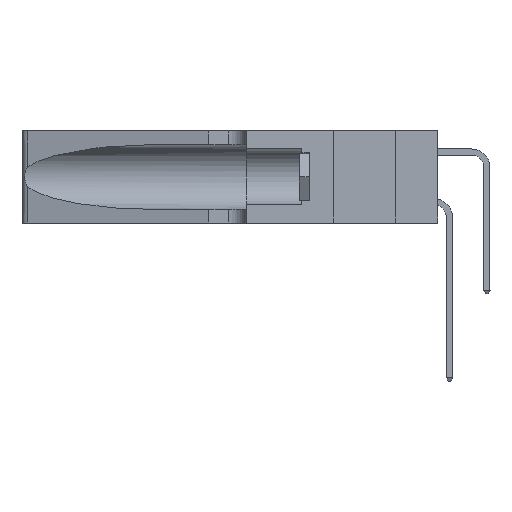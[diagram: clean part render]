
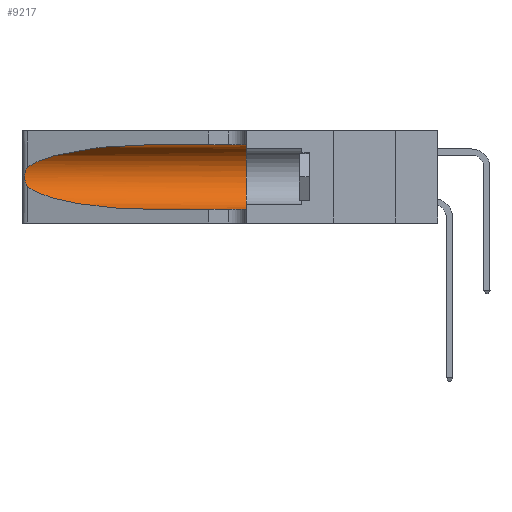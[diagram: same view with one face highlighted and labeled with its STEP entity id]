
A CAD part, left-side view. The second image highlights one B-rep face of the part: STEP entity #9217.
In plain terms, the highlighted cylindrical face has radius 3.308 mm (diameter 6.617 mm), a partial arc.
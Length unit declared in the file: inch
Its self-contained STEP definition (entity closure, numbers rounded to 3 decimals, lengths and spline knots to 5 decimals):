
#25 = VERTEX_POINT ( 'NONE', #38068 ) ;
#346 = CARTESIAN_POINT ( 'NONE',  ( 0.25487, 1.22718, 0.14631 ) ) ;
#667 = ORIENTED_EDGE ( 'NONE', *, *, #3955, .F. ) ;
#1703 = FACE_OUTER_BOUND ( 'NONE', #33231, .T. ) ;
#2833 = CARTESIAN_POINT ( 'NONE',  ( 0.25555, 1.22993, 0.14849 ) ) ;
#2927 = CARTESIAN_POINT ( 'NONE',  ( 0.2373, 1.15595, 0.08982 ) ) ;
#3357 = VERTEX_POINT ( 'NONE', #346 ) ;
#3804 = CARTESIAN_POINT ( 'NONE',  ( 0.1305, 0.72297, 0.05475 ) ) ;
#3955 = EDGE_CURVE ( 'NONE', #25, #28407, #20215, .T. ) ;
#4011 = ORIENTED_EDGE ( 'NONE', *, *, #23458, .T. ) ;
#5024 = CARTESIAN_POINT ( 'NONE',  ( 0.1305, 0.35, 0.05475 ) ) ;
#5117 = B_SPLINE_CURVE_WITH_KNOTS ( 'NONE', 3,
 ( #5623, #23829, #26789, #8834, #29805, #11863, #32823, #14911, #35775, #17950, #38713, #20964, #2833, #23957 ),
 .UNSPECIFIED., .F., .F.,
 ( 4, 2, 2, 2, 2, 2, 4 ),
 ( 0., 0.00027, 0.00053, 0.00107, 0.0016, 0.00187, 0.00214 ),
 .UNSPECIFIED. ) ;
#5476 = DIRECTION ( 'NONE',  ( 0., 0., -1. ) ) ;
#5623 = CARTESIAN_POINT ( 'NONE',  ( 0.25487, 1.22718, 0.22369 ) ) ;
#6643 = LINE ( 'NONE', #36633, #38463 ) ;
#6791 = EDGE_CURVE ( 'NONE', #25249, #28407, #6643, .T. ) ;
#7832 = CARTESIAN_POINT ( 'NONE',  ( 0.1305, 0.72297, 0.31525 ) ) ;
#8834 = CARTESIAN_POINT ( 'NONE',  ( 0.25787, 1.23484, 0.2124 ) ) ;
#9059 = CARTESIAN_POINT ( 'NONE',  ( 0.25487, 1.22718, 0.14631 ) ) ;
#9217 = ADVANCED_FACE ( 'NONE', ( #1703 ), #16909, .F. ) ;
#10066 = DIRECTION ( 'NONE',  ( 0., 1., 0. ) ) ;
#10710 = ORIENTED_EDGE ( 'NONE', *, *, #35669, .F. ) ;
#10867 = CARTESIAN_POINT ( 'NONE',  ( 0.2373, 1.15595, 0.28018 ) ) ;
#11863 = CARTESIAN_POINT ( 'NONE',  ( 0.26018, 1.23835, 0.19895 ) ) ;
#12324 = VECTOR ( 'NONE', #37208, 39.37008 ) ;
#12525 = CARTESIAN_POINT ( 'NONE',  ( 0.25487, 1.22718, 0.22369 ) ) ;
#13357 = CARTESIAN_POINT ( 'NONE',  ( 0.1305, 1.61858, 0.31525 ) ) ;
#14242 = LINE ( 'NONE', #13357, #12324 ) ;
#14911 = CARTESIAN_POINT ( 'NONE',  ( 0.26075, 1.23896, 0.178 ) ) ;
#14937 = EDGE_CURVE ( 'NONE', #23029, #3357, #5117, .T. ) ;
#16321 =( BOUNDED_CURVE ( )  B_SPLINE_CURVE ( 3, ( #7832, #28805, #10867, #31842 ),
 .UNSPECIFIED., .F., .F. ) 
 B_SPLINE_CURVE_WITH_KNOTS ( ( 4, 4 ),
 ( 1.5708, 2.84003 ),
 .UNSPECIFIED. ) 
 CURVE ( )  GEOMETRIC_REPRESENTATION_ITEM ( )  RATIONAL_B_SPLINE_CURVE ( ( 1., 0.87, 0.87, 1. ) ) 
 REPRESENTATION_ITEM ( '' )  );
#16909 = CYLINDRICAL_SURFACE ( 'NONE', #33762, 0.13025 ) ;
#17805 = CARTESIAN_POINT ( 'NONE',  ( 0.18966, 0.96281, 0.05475 ) ) ;
#17950 = CARTESIAN_POINT ( 'NONE',  ( 0.25856, 1.23593, 0.16098 ) ) ;
#18834 = DIRECTION ( 'NONE',  ( 0., -1., 0. ) ) ;
#20215 = CIRCLE ( 'NONE', #34363, 0.13025 ) ;
#20574 = DIRECTION ( 'NONE',  ( 0., -1., 0. ) ) ;
#20964 = CARTESIAN_POINT ( 'NONE',  ( 0.25639, 1.23186, 0.15144 ) ) ;
#21180 = CARTESIAN_POINT ( 'NONE',  ( 0.1305, 0.72297, 0.05475 ) ) ;
#21561 = CARTESIAN_POINT ( 'NONE',  ( 0.1305, 0.72297, 0.31525 ) ) ;
#21809 = VERTEX_POINT ( 'NONE', #21561 ) ;
#21999 = ORIENTED_EDGE ( 'NONE', *, *, #31473, .T. ) ;
#23029 = VERTEX_POINT ( 'NONE', #12525 ) ;
#23458 = EDGE_CURVE ( 'NONE', #21809, #23029, #16321, .T. ) ;
#23829 = CARTESIAN_POINT ( 'NONE',  ( 0.25555, 1.22994, 0.2215 ) ) ;
#23957 = CARTESIAN_POINT ( 'NONE',  ( 0.25487, 1.22718, 0.14631 ) ) ;
#25249 = VERTEX_POINT ( 'NONE', #3804 ) ;
#26789 = CARTESIAN_POINT ( 'NONE',  ( 0.25639, 1.23184, 0.21858 ) ) ;
#28000 = CARTESIAN_POINT ( 'NONE',  ( 0.1305, 0.35, 0.185 ) ) ;
#28027 = ORIENTED_EDGE ( 'NONE', *, *, #14937, .T. ) ;
#28407 = VERTEX_POINT ( 'NONE', #5024 ) ;
#28805 = CARTESIAN_POINT ( 'NONE',  ( 0.18966, 0.96281, 0.31525 ) ) ;
#29541 = CARTESIAN_POINT ( 'NONE',  ( 0.1305, 1.61858, 0.185 ) ) ;
#29805 = CARTESIAN_POINT ( 'NONE',  ( 0.25854, 1.2359, 0.20912 ) ) ;
#29916 = ORIENTED_EDGE ( 'NONE', *, *, #6791, .T. ) ;
#31053 = DIRECTION ( 'NONE',  ( 0., 0., 1. ) ) ;
#31473 = EDGE_CURVE ( 'NONE', #3357, #25249, #38216, .T. ) ;
#31842 = CARTESIAN_POINT ( 'NONE',  ( 0.25487, 1.22718, 0.22369 ) ) ;
#32823 = CARTESIAN_POINT ( 'NONE',  ( 0.26075, 1.23896, 0.19203 ) ) ;
#33231 = EDGE_LOOP ( 'NONE', ( #4011, #28027, #21999, #29916, #667, #10710 ) ) ;
#33762 = AXIS2_PLACEMENT_3D ( 'NONE', #29541, #20574, #5476 ) ;
#34363 = AXIS2_PLACEMENT_3D ( 'NONE', #28000, #10066, #31053 ) ;
#35669 = EDGE_CURVE ( 'NONE', #21809, #25, #14242, .T. ) ;
#35775 = CARTESIAN_POINT ( 'NONE',  ( 0.26017, 1.23833, 0.17102 ) ) ;
#36633 = CARTESIAN_POINT ( 'NONE',  ( 0.1305, 1.61858, 0.05475 ) ) ;
#37208 = DIRECTION ( 'NONE',  ( 0., -1., 0. ) ) ;
#38068 = CARTESIAN_POINT ( 'NONE',  ( 0.1305, 0.35, 0.31525 ) ) ;
#38216 =( BOUNDED_CURVE ( )  B_SPLINE_CURVE ( 3, ( #9059, #2927, #17805, #21180 ),
 .UNSPECIFIED., .F., .F. ) 
 B_SPLINE_CURVE_WITH_KNOTS ( ( 4, 4 ),
 ( 3.44316, 4.71239 ),
 .UNSPECIFIED. ) 
 CURVE ( )  GEOMETRIC_REPRESENTATION_ITEM ( )  RATIONAL_B_SPLINE_CURVE ( ( 1., 0.87, 0.87, 1. ) ) 
 REPRESENTATION_ITEM ( '' )  );
#38463 = VECTOR ( 'NONE', #18834, 39.37008 ) ;
#38713 = CARTESIAN_POINT ( 'NONE',  ( 0.25789, 1.23486, 0.15765 ) ) ;
